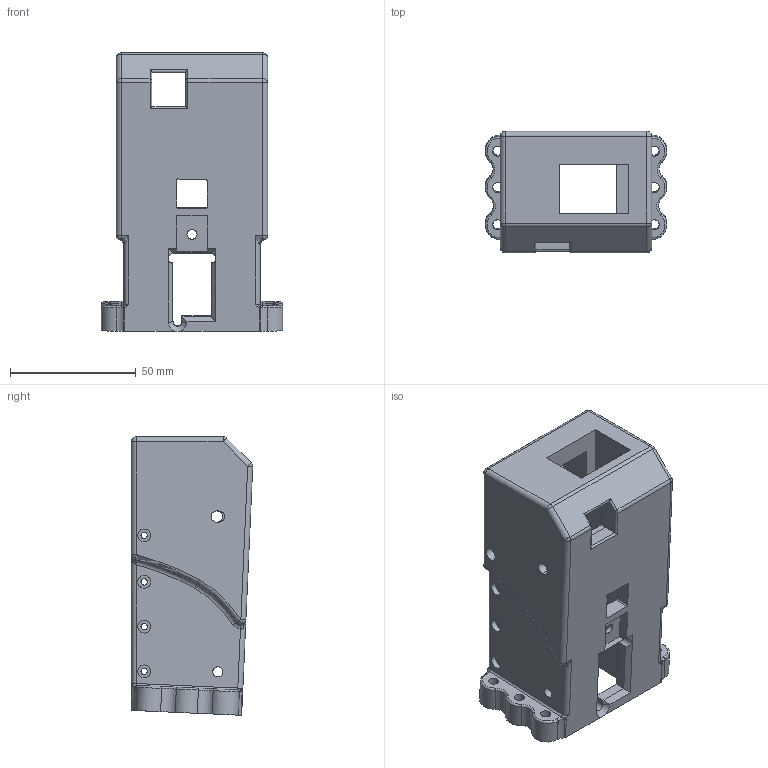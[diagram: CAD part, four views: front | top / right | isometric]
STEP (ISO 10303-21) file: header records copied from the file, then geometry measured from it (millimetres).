
FILE_DESCRIPTION(/* description */ (''),/* implementation_level */ '2;1');
FILE_NAME(/* name */ 'Plastikov v0.9 Rear Receiver.stp',/* time_stamp */ '2020-03-23T00:34:31-05:00',/* author */ ('johne'),/* organization */ (''),/* preprocessor_version */ 'ST-DEVELOPER v18',/* originating_system */ 'Autodesk Inventor 2020',/* authorisation */ '');
FILE_SCHEMA (('AUTOMOTIVE_DESIGN { 1 0 10303 214 3 1 1 }'));
Length unit declared in the file: millimetre
Products named in the file (1): Plastikov v0.9 Rear Receiver
Bounding box: 72.2 x 48.28 x 110.76 mm (x, y, z)
Volume: 148150.9 mm3; surface area: 38790.2 mm2
Topology: 1 solids, 1 shells, 223 faces, 588 edges, 367 vertices
Faces by surface type: cylinder 86, plane 69, torus 27, bspline 26, sphere 14, cone 1
Full cylindrical faces by diameter (mm): 2.5 x8, 3.12 x4, 4 x9, 4.5 x1, 5.08 x8
Entity records: 7963 total; most frequent: CARTESIAN_POINT 2263, DIRECTION 1225, ORIENTED_EDGE 1160, EDGE_CURVE 580, AXIS2_PLACEMENT_3D 488, VERTEX_POINT 367, EDGE_LOOP 277, CIRCLE 264
